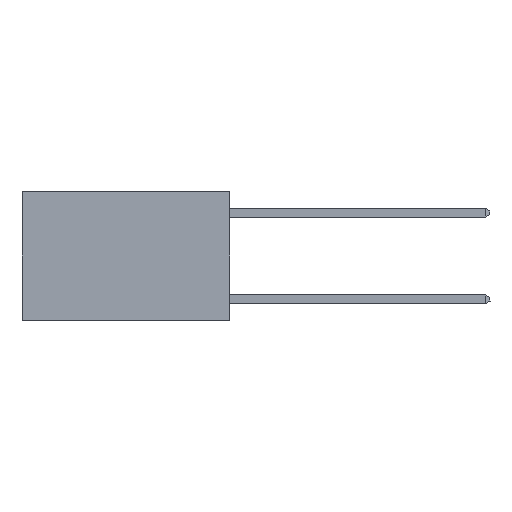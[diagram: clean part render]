
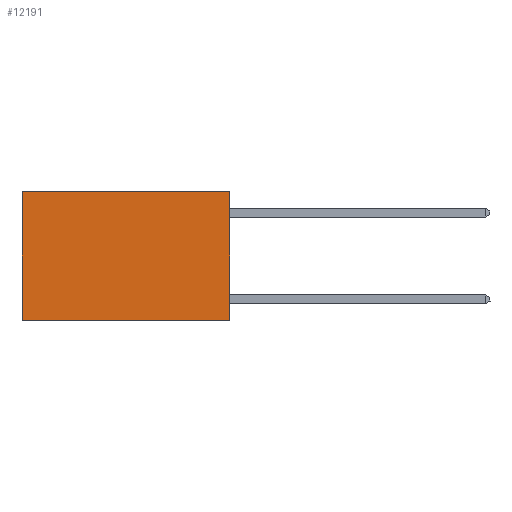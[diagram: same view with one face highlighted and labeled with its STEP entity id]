
A CAD part, left-side view. The second image highlights one B-rep face of the part: STEP entity #12191.
In plain terms, the highlighted planar face has unit normal (-1, 0, 0).
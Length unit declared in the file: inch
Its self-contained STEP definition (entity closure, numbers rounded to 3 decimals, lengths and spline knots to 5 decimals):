
#476 = PLANE ( 'NONE',  #16797 ) ;
#1225 = LINE ( 'NONE', #8022, #1779 ) ;
#1287 = ORIENTED_EDGE ( 'NONE', *, *, #19989, .T. ) ;
#1779 = VECTOR ( 'NONE', #16120, 39.37008 ) ;
#1820 = EDGE_LOOP ( 'NONE', ( #13434, #12145, #15229, #1287 ) ) ;
#2240 = EDGE_CURVE ( 'NONE', #8718, #16655, #1225, .T. ) ;
#2439 = FACE_OUTER_BOUND ( 'NONE', #1820, .T. ) ;
#3145 = LINE ( 'NONE', #4689, #7309 ) ;
#4033 = CARTESIAN_POINT ( 'NONE',  ( 0.2625, 0., 0. ) ) ;
#4689 = CARTESIAN_POINT ( 'NONE',  ( 0.2625, 0., 0. ) ) ;
#5807 = DIRECTION ( 'NONE',  ( 0., 0., -1. ) ) ;
#5947 = CARTESIAN_POINT ( 'NONE',  ( 0.2625, 0.6, 0. ) ) ;
#6501 = CARTESIAN_POINT ( 'NONE',  ( 0.2625, 0.6, 0. ) ) ;
#7309 = VECTOR ( 'NONE', #8360, 39.37008 ) ;
#8022 = CARTESIAN_POINT ( 'NONE',  ( 0.2625, 0., -0.37 ) ) ;
#8237 = LINE ( 'NONE', #22174, #21454 ) ;
#8327 = DIRECTION ( 'NONE',  ( 0., 0., -1. ) ) ;
#8360 = DIRECTION ( 'NONE',  ( 0., 0., -1. ) ) ;
#8718 = VERTEX_POINT ( 'NONE', #11051 ) ;
#9906 = LINE ( 'NONE', #6501, #13977 ) ;
#10909 = VERTEX_POINT ( 'NONE', #5947 ) ;
#11051 = CARTESIAN_POINT ( 'NONE',  ( 0.2625, 0., -0.37 ) ) ;
#11376 = CARTESIAN_POINT ( 'NONE',  ( 0.2625, 0., 0. ) ) ;
#12145 = ORIENTED_EDGE ( 'NONE', *, *, #2240, .F. ) ;
#12191 = ADVANCED_FACE ( 'NONE', ( #2439 ), #476, .F. ) ;
#12483 = EDGE_CURVE ( 'NONE', #10909, #16655, #9906, .T. ) ;
#13434 = ORIENTED_EDGE ( 'NONE', *, *, #12483, .T. ) ;
#13693 = DIRECTION ( 'NONE',  ( 0., 1., 0. ) ) ;
#13977 = VECTOR ( 'NONE', #8327, 39.37008 ) ;
#15229 = ORIENTED_EDGE ( 'NONE', *, *, #15322, .F. ) ;
#15322 = EDGE_CURVE ( 'NONE', #16082, #8718, #3145, .T. ) ;
#16082 = VERTEX_POINT ( 'NONE', #11376 ) ;
#16120 = DIRECTION ( 'NONE',  ( 0., 1., 0. ) ) ;
#16341 = DIRECTION ( 'NONE',  ( 1., 0., 0. ) ) ;
#16655 = VERTEX_POINT ( 'NONE', #18390 ) ;
#16797 = AXIS2_PLACEMENT_3D ( 'NONE', #4033, #16341, #5807 ) ;
#18390 = CARTESIAN_POINT ( 'NONE',  ( 0.2625, 0.6, -0.37 ) ) ;
#19989 = EDGE_CURVE ( 'NONE', #16082, #10909, #8237, .T. ) ;
#21454 = VECTOR ( 'NONE', #13693, 39.37008 ) ;
#22174 = CARTESIAN_POINT ( 'NONE',  ( 0.2625, 0., 0. ) ) ;
